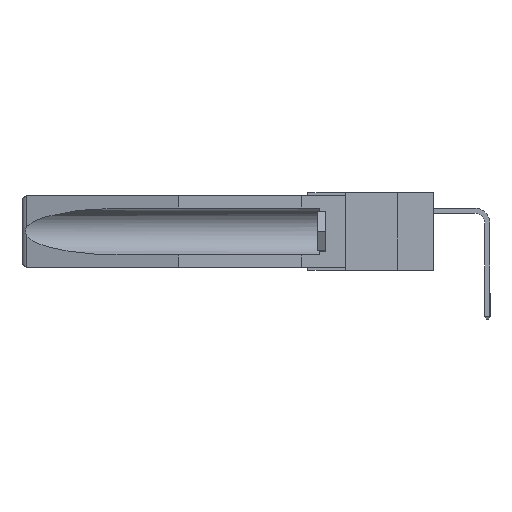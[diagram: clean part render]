
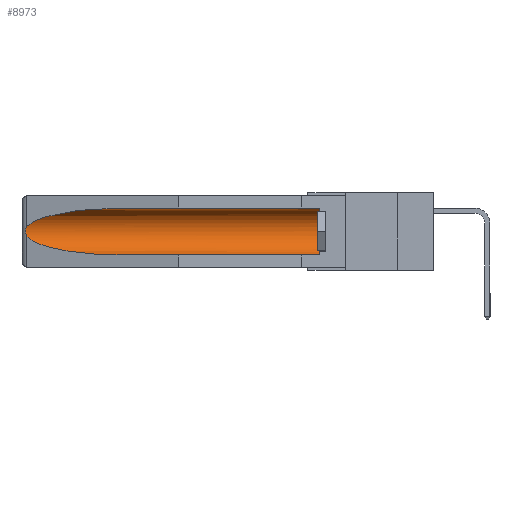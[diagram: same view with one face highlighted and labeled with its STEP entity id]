
A CAD part, left-side view. The second image highlights one B-rep face of the part: STEP entity #8973.
In plain terms, the highlighted cylindrical face has radius 2.857 mm (diameter 5.715 mm), a partial arc.
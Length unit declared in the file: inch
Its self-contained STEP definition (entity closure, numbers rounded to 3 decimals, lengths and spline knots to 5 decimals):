
#121 = CARTESIAN_POINT ( 'NONE',  ( 0.26537, 1.52718, -0.19328 ) ) ;
#249 = LINE ( 'NONE', #20942, #11374 ) ;
#447 = VERTEX_POINT ( 'NONE', #26508 ) ;
#1197 = CARTESIAN_POINT ( 'NONE',  ( 0.26537, 1.52718, -0.19328 ) ) ;
#1777 =( BOUNDED_CURVE ( )  B_SPLINE_CURVE ( 3, ( #19855, #10883, #6116, #3717 ),
 .UNSPECIFIED., .F., .F. ) 
 B_SPLINE_CURVE_WITH_KNOTS ( ( 4, 4 ),
 ( 4.71239, 6.08839 ),
 .UNSPECIFIED. ) 
 CURVE ( )  GEOMETRIC_REPRESENTATION_ITEM ( )  RATIONAL_B_SPLINE_CURVE ( ( 1., 0.848, 0.848, 1. ) ) 
 REPRESENTATION_ITEM ( '' )  );
#1832 = DIRECTION ( 'NONE',  ( 0., 1., 0. ) ) ;
#1870 = DIRECTION ( 'NONE',  ( 0., -1., 0. ) ) ;
#1910 = CARTESIAN_POINT ( 'NONE',  ( 0.2673, 1.53269, -0.17917 ) ) ;
#2089 = CARTESIAN_POINT ( 'NONE',  ( 0.155, 0.126, -0.284 ) ) ;
#2394 = FACE_OUTER_BOUND ( 'NONE', #17343, .T. ) ;
#3717 = CARTESIAN_POINT ( 'NONE',  ( 0.26537, 1.52718, -0.14972 ) ) ;
#3969 = CARTESIAN_POINT ( 'NONE',  ( 0.2675, 1.53308, -0.16763 ) ) ;
#4040 = AXIS2_PLACEMENT_3D ( 'NONE', #8661, #1832, #20134 ) ;
#4076 = CARTESIAN_POINT ( 'NONE',  ( 0.26655, 1.53094, -0.18657 ) ) ;
#4529 = DIRECTION ( 'NONE',  ( 0., 0., 1. ) ) ;
#6116 = CARTESIAN_POINT ( 'NONE',  ( 0.25451, 1.48313, -0.09465 ) ) ;
#6208 = ORIENTED_EDGE ( 'NONE', *, *, #27835, .T. ) ;
#6243 = CARTESIAN_POINT ( 'NONE',  ( 0.21114, 1.30732, -0.284 ) ) ;
#6472 = CARTESIAN_POINT ( 'NONE',  ( 0.26537, 1.52718, -0.14972 ) ) ;
#7398 = LINE ( 'NONE', #20262, #25240 ) ;
#8637 = CARTESIAN_POINT ( 'NONE',  ( 0.2673, 1.5327, -0.16383 ) ) ;
#8661 = CARTESIAN_POINT ( 'NONE',  ( 0.155, -0.30754, -0.1715 ) ) ;
#8973 = ADVANCED_FACE ( 'NONE', ( #2394 ), #13142, .F. ) ;
#9990 = ORIENTED_EDGE ( 'NONE', *, *, #28987, .T. ) ;
#10255 = ORIENTED_EDGE ( 'NONE', *, *, #19379, .F. ) ;
#10883 = CARTESIAN_POINT ( 'NONE',  ( 0.21114, 1.30732, -0.059 ) ) ;
#11241 = AXIS2_PLACEMENT_3D ( 'NONE', #13315, #1870, #4529 ) ;
#11374 = VECTOR ( 'NONE', #25230, 39.37008 ) ;
#11537 =( BOUNDED_CURVE ( )  B_SPLINE_CURVE ( 3, ( #1197, #17496, #6243, #13232 ),
 .UNSPECIFIED., .F., .F. ) 
 B_SPLINE_CURVE_WITH_KNOTS ( ( 4, 4 ),
 ( 0.1948, 1.5708 ),
 .UNSPECIFIED. ) 
 CURVE ( )  GEOMETRIC_REPRESENTATION_ITEM ( )  RATIONAL_B_SPLINE_CURVE ( ( 1., 0.848, 0.848, 1. ) ) 
 REPRESENTATION_ITEM ( '' )  );
#12854 = CIRCLE ( 'NONE', #11241, 0.1125 ) ;
#13142 = CYLINDRICAL_SURFACE ( 'NONE', #4040, 0.1125 ) ;
#13194 = ORIENTED_EDGE ( 'NONE', *, *, #20401, .T. ) ;
#13232 = CARTESIAN_POINT ( 'NONE',  ( 0.155, 1.07973, -0.284 ) ) ;
#13315 = CARTESIAN_POINT ( 'NONE',  ( 0.155, 0.126, -0.1715 ) ) ;
#17318 = CARTESIAN_POINT ( 'NONE',  ( 0.155, 1.07973, -0.284 ) ) ;
#17343 = EDGE_LOOP ( 'NONE', ( #18608, #9990, #22554, #10255, #6208, #13194 ) ) ;
#17430 = VERTEX_POINT ( 'NONE', #17318 ) ;
#17496 = CARTESIAN_POINT ( 'NONE',  ( 0.25451, 1.48313, -0.24835 ) ) ;
#17716 = CARTESIAN_POINT ( 'NONE',  ( 0.26597, 1.52961, -0.15275 ) ) ;
#17905 = VERTEX_POINT ( 'NONE', #2089 ) ;
#18311 = VERTEX_POINT ( 'NONE', #28810 ) ;
#18608 = ORIENTED_EDGE ( 'NONE', *, *, #25691, .T. ) ;
#19379 = EDGE_CURVE ( 'NONE', #17905, #17430, #249, .T. ) ;
#19703 = VERTEX_POINT ( 'NONE', #24297 ) ;
#19855 = CARTESIAN_POINT ( 'NONE',  ( 0.155, 1.07973, -0.059 ) ) ;
#19901 = CARTESIAN_POINT ( 'NONE',  ( 0.2675, 1.53308, -0.17534 ) ) ;
#20134 = DIRECTION ( 'NONE',  ( 0., 0., 1. ) ) ;
#20262 = CARTESIAN_POINT ( 'NONE',  ( 0.155, -0.30754, -0.059 ) ) ;
#20401 = EDGE_CURVE ( 'NONE', #18311, #19703, #7398, .T. ) ;
#20942 = CARTESIAN_POINT ( 'NONE',  ( 0.155, -0.30754, -0.284 ) ) ;
#21221 = B_SPLINE_CURVE_WITH_KNOTS ( 'NONE', 3,
 ( #6472, #17716, #24700, #8637, #3969, #19901, #1910, #4076, #26793, #22194 ),
 .UNSPECIFIED., .F., .F.,
 ( 4, 2, 2, 2, 4 ),
 ( 0., 0.00029, 0.00058, 0.00087, 0.00117 ),
 .UNSPECIFIED. ) ;
#22194 = CARTESIAN_POINT ( 'NONE',  ( 0.26537, 1.52718, -0.19328 ) ) ;
#22554 = ORIENTED_EDGE ( 'NONE', *, *, #23057, .T. ) ;
#23057 = EDGE_CURVE ( 'NONE', #26556, #17430, #11537, .T. ) ;
#24297 = CARTESIAN_POINT ( 'NONE',  ( 0.155, 1.07973, -0.059 ) ) ;
#24700 = CARTESIAN_POINT ( 'NONE',  ( 0.26654, 1.53092, -0.15636 ) ) ;
#25230 = DIRECTION ( 'NONE',  ( 0., 1., 0. ) ) ;
#25240 = VECTOR ( 'NONE', #27159, 39.37008 ) ;
#25691 = EDGE_CURVE ( 'NONE', #19703, #447, #1777, .T. ) ;
#26508 = CARTESIAN_POINT ( 'NONE',  ( 0.26537, 1.52718, -0.14972 ) ) ;
#26556 = VERTEX_POINT ( 'NONE', #121 ) ;
#26793 = CARTESIAN_POINT ( 'NONE',  ( 0.26597, 1.5296, -0.19026 ) ) ;
#27159 = DIRECTION ( 'NONE',  ( 0., 1., 0. ) ) ;
#27835 = EDGE_CURVE ( 'NONE', #17905, #18311, #12854, .T. ) ;
#28810 = CARTESIAN_POINT ( 'NONE',  ( 0.155, 0.126, -0.059 ) ) ;
#28987 = EDGE_CURVE ( 'NONE', #447, #26556, #21221, .T. ) ;
